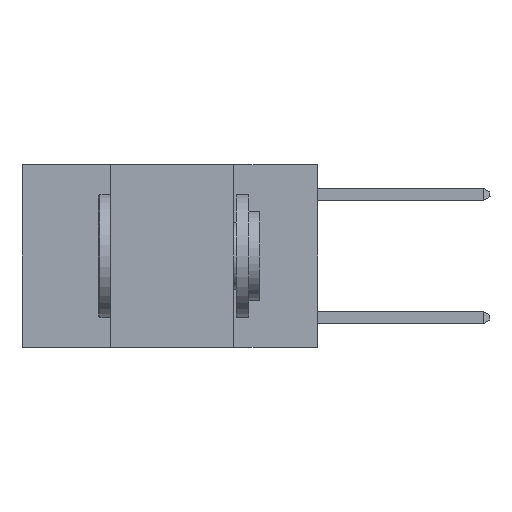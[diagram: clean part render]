
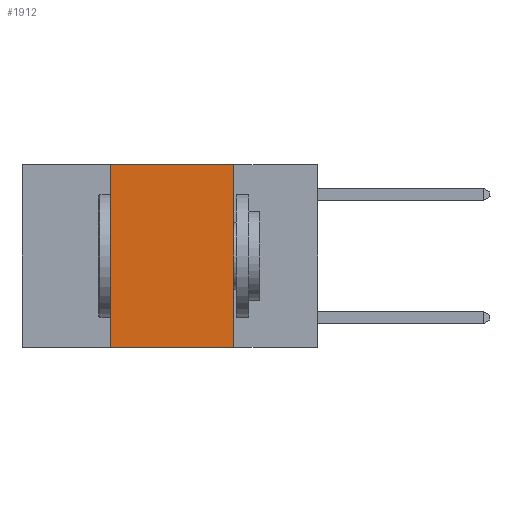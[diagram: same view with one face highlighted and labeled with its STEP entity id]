
A CAD part, left-side view. The second image highlights one B-rep face of the part: STEP entity #1912.
In plain terms, the highlighted planar face has unit normal (-1, 0, 0).
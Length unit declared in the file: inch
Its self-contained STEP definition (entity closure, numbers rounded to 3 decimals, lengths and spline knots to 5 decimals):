
#87 = CARTESIAN_POINT ( 'NONE',  ( 0., 0.17, -0.37 ) ) ;
#113 = CARTESIAN_POINT ( 'NONE',  ( 0., 0.6, 0. ) ) ;
#705 = ORIENTED_EDGE ( 'NONE', *, *, #1512, .F. ) ;
#1337 = CARTESIAN_POINT ( 'NONE',  ( 0., 0.42, -0.37 ) ) ;
#1364 = VECTOR ( 'NONE', #8134, 39.37008 ) ;
#1512 = EDGE_CURVE ( 'NONE', #3937, #3746, #4339, .T. ) ;
#1912 = ADVANCED_FACE ( 'NONE', ( #2641 ), #7786, .F. ) ;
#2160 = AXIS2_PLACEMENT_3D ( 'NONE', #5258, #6786, #5249 ) ;
#2527 = VECTOR ( 'NONE', #5043, 39.37008 ) ;
#2641 = FACE_OUTER_BOUND ( 'NONE', #3675, .T. ) ;
#2712 = VECTOR ( 'NONE', #6131, 39.37008 ) ;
#2819 = CARTESIAN_POINT ( 'NONE',  ( 0., 0.17, 0. ) ) ;
#3675 = EDGE_LOOP ( 'NONE', ( #4409, #6441, #705, #6641 ) ) ;
#3746 = VERTEX_POINT ( 'NONE', #3961 ) ;
#3937 = VERTEX_POINT ( 'NONE', #1337 ) ;
#3961 = CARTESIAN_POINT ( 'NONE',  ( 0., 0.42, 0. ) ) ;
#4339 = LINE ( 'NONE', #7057, #2527 ) ;
#4409 = ORIENTED_EDGE ( 'NONE', *, *, #6922, .F. ) ;
#4492 = EDGE_CURVE ( 'NONE', #3937, #5586, #8782, .T. ) ;
#4628 = EDGE_CURVE ( 'NONE', #3746, #9908, #5621, .T. ) ;
#5043 = DIRECTION ( 'NONE',  ( 0., 0., 1. ) ) ;
#5249 = DIRECTION ( 'NONE',  ( 0., 0., -1. ) ) ;
#5258 = CARTESIAN_POINT ( 'NONE',  ( 0., 0.6, 0. ) ) ;
#5375 = CARTESIAN_POINT ( 'NONE',  ( 0., 0.6, -0.37 ) ) ;
#5381 = VECTOR ( 'NONE', #8549, 39.37008 ) ;
#5586 = VERTEX_POINT ( 'NONE', #87 ) ;
#5621 = LINE ( 'NONE', #113, #5381 ) ;
#5706 = LINE ( 'NONE', #2819, #1364 ) ;
#6131 = DIRECTION ( 'NONE',  ( 0., -1., 0. ) ) ;
#6441 = ORIENTED_EDGE ( 'NONE', *, *, #4628, .F. ) ;
#6641 = ORIENTED_EDGE ( 'NONE', *, *, #4492, .T. ) ;
#6786 = DIRECTION ( 'NONE',  ( 1., 0., 0. ) ) ;
#6922 = EDGE_CURVE ( 'NONE', #9908, #5586, #5706, .T. ) ;
#7057 = CARTESIAN_POINT ( 'NONE',  ( 0., 0.42, 0. ) ) ;
#7786 = PLANE ( 'NONE',  #2160 ) ;
#8134 = DIRECTION ( 'NONE',  ( 0., 0., -1. ) ) ;
#8549 = DIRECTION ( 'NONE',  ( 0., -1., 0. ) ) ;
#8782 = LINE ( 'NONE', #5375, #2712 ) ;
#9434 = CARTESIAN_POINT ( 'NONE',  ( 0., 0.17, 0. ) ) ;
#9908 = VERTEX_POINT ( 'NONE', #9434 ) ;
